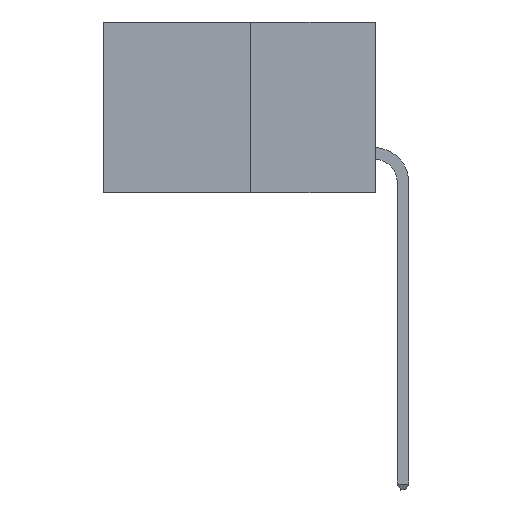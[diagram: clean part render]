
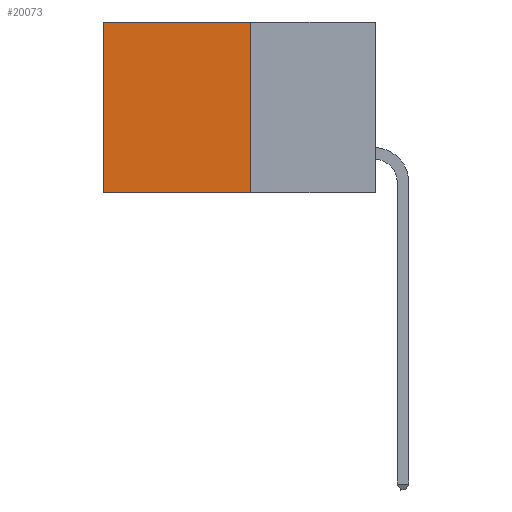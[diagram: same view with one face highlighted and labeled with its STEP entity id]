
A CAD part, left-side view. The second image highlights one B-rep face of the part: STEP entity #20073.
In plain terms, the highlighted planar face has unit normal (-1, 0, 0).
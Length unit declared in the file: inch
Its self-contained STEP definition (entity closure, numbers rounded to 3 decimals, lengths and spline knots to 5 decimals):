
#256 = EDGE_CURVE ( 'NONE', #8128, #27776, #28524, .T. ) ;
#2119 = DIRECTION ( 'NONE',  ( 1., 0., 0. ) ) ;
#2661 = VECTOR ( 'NONE', #8478, 39.37008 ) ;
#3436 = ORIENTED_EDGE ( 'NONE', *, *, #256, .T. ) ;
#3567 = DIRECTION ( 'NONE',  ( 0., 0., -1. ) ) ;
#3675 = CARTESIAN_POINT ( 'NONE',  ( 0.277, 0.27, -0.37 ) ) ;
#3965 = EDGE_CURVE ( 'NONE', #26458, #8128, #19668, .T. ) ;
#4298 = ORIENTED_EDGE ( 'NONE', *, *, #9593, .F. ) ;
#4768 = EDGE_CURVE ( 'NONE', #18121, #27776, #21830, .T. ) ;
#4925 = CARTESIAN_POINT ( 'NONE',  ( 0.277, 0.27, -0.37 ) ) ;
#6607 = VECTOR ( 'NONE', #21680, 39.37008 ) ;
#7520 = AXIS2_PLACEMENT_3D ( 'NONE', #23976, #2119, #19245 ) ;
#8128 = VERTEX_POINT ( 'NONE', #23678 ) ;
#8478 = DIRECTION ( 'NONE',  ( 0., 0., -1. ) ) ;
#9593 = EDGE_CURVE ( 'NONE', #26458, #18121, #11585, .T. ) ;
#11585 = LINE ( 'NONE', #3675, #23747 ) ;
#11862 = PLANE ( 'NONE',  #7520 ) ;
#12521 = ORIENTED_EDGE ( 'NONE', *, *, #4768, .F. ) ;
#14566 = EDGE_LOOP ( 'NONE', ( #3436, #12521, #4298, #15985 ) ) ;
#15985 = ORIENTED_EDGE ( 'NONE', *, *, #3965, .T. ) ;
#18121 = VERTEX_POINT ( 'NONE', #4925 ) ;
#19245 = DIRECTION ( 'NONE',  ( 0., 0., -1. ) ) ;
#19668 = LINE ( 'NONE', #22361, #6607 ) ;
#20073 = ADVANCED_FACE ( 'NONE', ( #28938 ), #11862, .F. ) ;
#21104 = VECTOR ( 'NONE', #29137, 39.37008 ) ;
#21680 = DIRECTION ( 'NONE',  ( 0., 1., 0. ) ) ;
#21830 = LINE ( 'NONE', #28936, #21104 ) ;
#21943 = CARTESIAN_POINT ( 'NONE',  ( 0.277, 0.59, -0.37 ) ) ;
#22361 = CARTESIAN_POINT ( 'NONE',  ( 0.277, 0.27, 0. ) ) ;
#23678 = CARTESIAN_POINT ( 'NONE',  ( 0.277, 0.59, 0. ) ) ;
#23747 = VECTOR ( 'NONE', #3567, 39.37008 ) ;
#23976 = CARTESIAN_POINT ( 'NONE',  ( 0.277, 0.27, -0.37 ) ) ;
#24654 = CARTESIAN_POINT ( 'NONE',  ( 0.277, 0.59, -0.37 ) ) ;
#26458 = VERTEX_POINT ( 'NONE', #31417 ) ;
#27776 = VERTEX_POINT ( 'NONE', #21943 ) ;
#28524 = LINE ( 'NONE', #24654, #2661 ) ;
#28936 = CARTESIAN_POINT ( 'NONE',  ( 0.277, 0.27, -0.37 ) ) ;
#28938 = FACE_OUTER_BOUND ( 'NONE', #14566, .T. ) ;
#29137 = DIRECTION ( 'NONE',  ( 0., 1., 0. ) ) ;
#31417 = CARTESIAN_POINT ( 'NONE',  ( 0.277, 0.27, 0. ) ) ;
